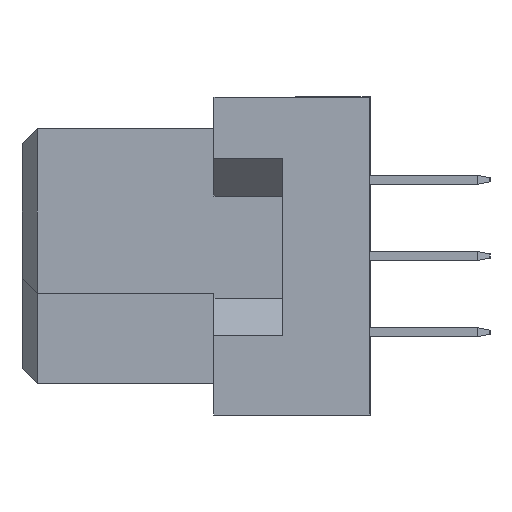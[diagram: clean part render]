
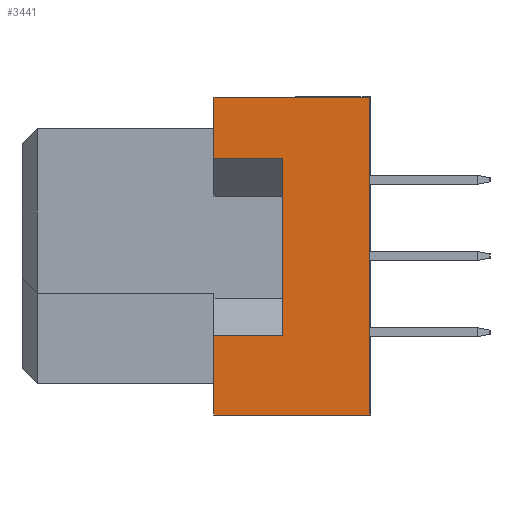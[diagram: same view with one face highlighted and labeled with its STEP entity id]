
A CAD part, left-side view. The second image highlights one B-rep face of the part: STEP entity #3441.
In plain terms, the highlighted planar face has unit normal (-1, 0, 0).
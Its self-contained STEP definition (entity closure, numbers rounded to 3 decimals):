
#66 = VERTEX_POINT ( 'NONE', #20224 ) ;
#663 = LINE ( 'NONE', #9804, #24914 ) ;
#696 = LINE ( 'NONE', #36453, #33151 ) ;
#1452 = CARTESIAN_POINT ( 'NONE',  ( -47.5, -11.6, 5.3 ) ) ;
#3285 = EDGE_CURVE ( 'NONE', #13466, #66, #696, .T. ) ;
#3345 = AXIS2_PLACEMENT_3D ( 'NONE', #22525, #28673, #10625 ) ;
#3441 = ADVANCED_FACE ( 'NONE', ( #16369 ), #10429, .T. ) ;
#3527 = DIRECTION ( 'NONE',  ( 0., 1., 0. ) ) ;
#3749 = EDGE_LOOP ( 'NONE', ( #20639, #39054, #37952, #11354, #38082, #20580, #20187, #3954 ) ) ;
#3826 = CARTESIAN_POINT ( 'NONE',  ( -47.5, -11.6, 5.3 ) ) ;
#3954 = ORIENTED_EDGE ( 'NONE', *, *, #4730, .F. ) ;
#4730 = EDGE_CURVE ( 'NONE', #15276, #9685, #663, .T. ) ;
#5501 = VECTOR ( 'NONE', #7949, 1000. ) ;
#5896 = VECTOR ( 'NONE', #8609, 1000. ) ;
#6306 = CARTESIAN_POINT ( 'NONE',  ( -47.5, -8.7, 3.25 ) ) ;
#6512 = CARTESIAN_POINT ( 'NONE',  ( -47.5, -8.7, -2.65 ) ) ;
#6790 = CARTESIAN_POINT ( 'NONE',  ( -47.5, -6.4, -5.3 ) ) ;
#7949 = DIRECTION ( 'NONE',  ( 0., 1., 0. ) ) ;
#8609 = DIRECTION ( 'NONE',  ( 0., 1., 0. ) ) ;
#9685 = VERTEX_POINT ( 'NONE', #6306 ) ;
#9804 = CARTESIAN_POINT ( 'NONE',  ( -47.5, -8.7, -2.65 ) ) ;
#10325 = VERTEX_POINT ( 'NONE', #32239 ) ;
#10429 = PLANE ( 'NONE',  #3345 ) ;
#10625 = DIRECTION ( 'NONE',  ( 0., 0., 1. ) ) ;
#10820 = EDGE_CURVE ( 'NONE', #14432, #28120, #15049, .T. ) ;
#11354 = ORIENTED_EDGE ( 'NONE', *, *, #33002, .T. ) ;
#12240 = CARTESIAN_POINT ( 'NONE',  ( -47.5, -11.6, -5.3 ) ) ;
#13466 = VERTEX_POINT ( 'NONE', #17309 ) ;
#14432 = VERTEX_POINT ( 'NONE', #12240 ) ;
#14808 = DIRECTION ( 'NONE',  ( 0., 0., 1. ) ) ;
#15049 = LINE ( 'NONE', #33514, #29563 ) ;
#15276 = VERTEX_POINT ( 'NONE', #15453 ) ;
#15453 = CARTESIAN_POINT ( 'NONE',  ( -47.5, -8.7, -2.65 ) ) ;
#16369 = FACE_OUTER_BOUND ( 'NONE', #3749, .T. ) ;
#17309 = CARTESIAN_POINT ( 'NONE',  ( -47.5, -6.4, 3.25 ) ) ;
#18732 = DIRECTION ( 'NONE',  ( 0., 0., 1. ) ) ;
#19396 = EDGE_CURVE ( 'NONE', #15276, #10325, #33706, .T. ) ;
#19850 = LINE ( 'NONE', #25609, #5501 ) ;
#20166 = CARTESIAN_POINT ( 'NONE',  ( -47.5, -6.4, -5.3 ) ) ;
#20187 = ORIENTED_EDGE ( 'NONE', *, *, #37330, .F. ) ;
#20224 = CARTESIAN_POINT ( 'NONE',  ( -47.5, -6.4, 5.3 ) ) ;
#20438 = VECTOR ( 'NONE', #14808, 1000. ) ;
#20580 = ORIENTED_EDGE ( 'NONE', *, *, #3285, .F. ) ;
#20639 = ORIENTED_EDGE ( 'NONE', *, *, #19396, .T. ) ;
#21632 = EDGE_CURVE ( 'NONE', #34755, #66, #22505, .T. ) ;
#21871 = LINE ( 'NONE', #6790, #33036 ) ;
#22505 = LINE ( 'NONE', #1452, #5896 ) ;
#22525 = CARTESIAN_POINT ( 'NONE',  ( -47.5, -11.6, 5.3 ) ) ;
#23542 = CARTESIAN_POINT ( 'NONE',  ( -47.5, -11.6, 5.3 ) ) ;
#24129 = LINE ( 'NONE', #23542, #20438 ) ;
#24914 = VECTOR ( 'NONE', #18732, 1000. ) ;
#25609 = CARTESIAN_POINT ( 'NONE',  ( -47.5, -8.7, 3.25 ) ) ;
#28120 = VERTEX_POINT ( 'NONE', #20166 ) ;
#28673 = DIRECTION ( 'NONE',  ( -1., 0., 0. ) ) ;
#29563 = VECTOR ( 'NONE', #30712, 1000. ) ;
#30712 = DIRECTION ( 'NONE',  ( 0., 1., 0. ) ) ;
#30899 = EDGE_CURVE ( 'NONE', #28120, #10325, #21871, .T. ) ;
#32239 = CARTESIAN_POINT ( 'NONE',  ( -47.5, -6.4, -2.65 ) ) ;
#33002 = EDGE_CURVE ( 'NONE', #14432, #34755, #24129, .T. ) ;
#33036 = VECTOR ( 'NONE', #37545, 1000. ) ;
#33151 = VECTOR ( 'NONE', #36836, 1000. ) ;
#33514 = CARTESIAN_POINT ( 'NONE',  ( -47.5, -11.6, -5.3 ) ) ;
#33706 = LINE ( 'NONE', #6512, #35174 ) ;
#34755 = VERTEX_POINT ( 'NONE', #3826 ) ;
#35174 = VECTOR ( 'NONE', #3527, 1000. ) ;
#36453 = CARTESIAN_POINT ( 'NONE',  ( -47.5, -6.4, -5.3 ) ) ;
#36836 = DIRECTION ( 'NONE',  ( 0., 0., 1. ) ) ;
#37330 = EDGE_CURVE ( 'NONE', #9685, #13466, #19850, .T. ) ;
#37545 = DIRECTION ( 'NONE',  ( 0., 0., 1. ) ) ;
#37952 = ORIENTED_EDGE ( 'NONE', *, *, #10820, .F. ) ;
#38082 = ORIENTED_EDGE ( 'NONE', *, *, #21632, .T. ) ;
#39054 = ORIENTED_EDGE ( 'NONE', *, *, #30899, .F. ) ;
